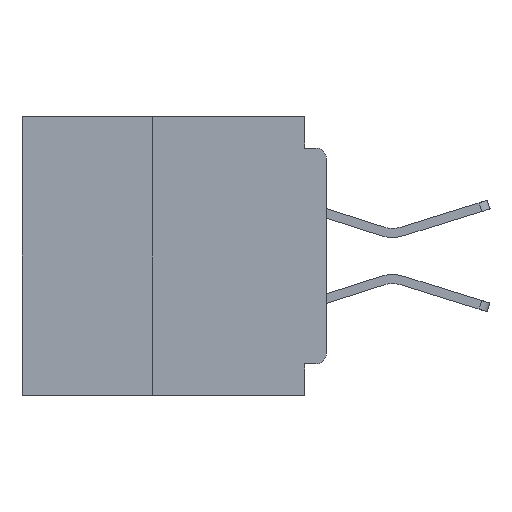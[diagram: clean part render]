
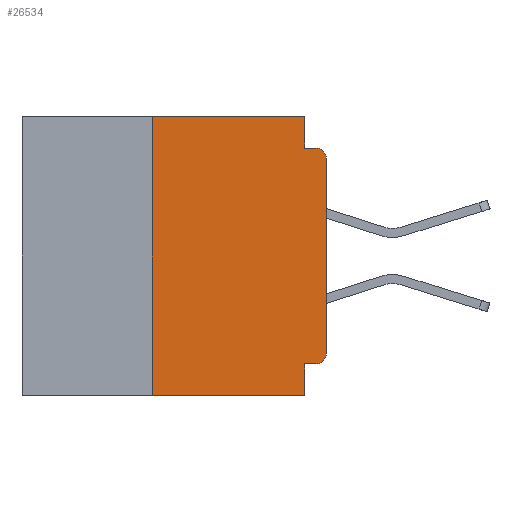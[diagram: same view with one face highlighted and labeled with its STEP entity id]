
A CAD part, left-side view. The second image highlights one B-rep face of the part: STEP entity #26534.
In plain terms, the highlighted planar face has unit normal (-1, 0, 0).
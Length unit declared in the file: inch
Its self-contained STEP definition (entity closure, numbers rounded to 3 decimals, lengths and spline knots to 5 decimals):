
#255 = CARTESIAN_POINT ( 'NONE',  ( 0., 0.437, -0.4 ) ) ;
#380 = AXIS2_PLACEMENT_3D ( 'NONE', #38324, #18297, #41635 ) ;
#1920 = ORIENTED_EDGE ( 'NONE', *, *, #42422, .T. ) ;
#1972 = VECTOR ( 'NONE', #17697, 39.37008 ) ;
#2018 = ORIENTED_EDGE ( 'NONE', *, *, #5475, .F. ) ;
#2225 = CIRCLE ( 'NONE', #36719, 0.015 ) ;
#2413 = EDGE_CURVE ( 'NONE', #28205, #35702, #32379, .T. ) ;
#3160 = CARTESIAN_POINT ( 'NONE',  ( 0., 0.015, -0.045 ) ) ;
#3316 = CARTESIAN_POINT ( 'NONE',  ( 0., 0.015, -0.34 ) ) ;
#3603 = CARTESIAN_POINT ( 'NONE',  ( 0., 0.031, -0.045 ) ) ;
#4029 = VECTOR ( 'NONE', #32181, 39.37008 ) ;
#4201 = VECTOR ( 'NONE', #35936, 39.37008 ) ;
#4441 = VECTOR ( 'NONE', #23019, 39.37008 ) ;
#4959 = CARTESIAN_POINT ( 'NONE',  ( 0., 0.25, -0.4 ) ) ;
#5108 = DIRECTION ( 'NONE',  ( 0., 0., 1. ) ) ;
#5475 = EDGE_CURVE ( 'NONE', #24682, #28205, #11640, .T. ) ;
#5590 = EDGE_CURVE ( 'NONE', #29763, #23510, #11081, .T. ) ;
#5641 = CARTESIAN_POINT ( 'NONE',  ( 0., 0., 0. ) ) ;
#6730 = DIRECTION ( 'NONE',  ( 0., 0., -1. ) ) ;
#7589 = EDGE_CURVE ( 'NONE', #35250, #29763, #30915, .T. ) ;
#7740 = LINE ( 'NONE', #255, #26707 ) ;
#8879 = CARTESIAN_POINT ( 'NONE',  ( 0., 0.437, 0. ) ) ;
#10181 = DIRECTION ( 'NONE',  ( 0., -1., 0. ) ) ;
#10432 = DIRECTION ( 'NONE',  ( 0., -1., 0. ) ) ;
#11081 = LINE ( 'NONE', #34374, #1972 ) ;
#11315 = AXIS2_PLACEMENT_3D ( 'NONE', #8879, #35766, #15731 ) ;
#11640 = LINE ( 'NONE', #20490, #16378 ) ;
#12328 = PLANE ( 'NONE',  #11315 ) ;
#12780 = CIRCLE ( 'NONE', #380, 0.015 ) ;
#13079 = EDGE_CURVE ( 'NONE', #35702, #27366, #16376, .T. ) ;
#13273 = LINE ( 'NONE', #5641, #4201 ) ;
#14278 = CARTESIAN_POINT ( 'NONE',  ( 0., 0.031, 0. ) ) ;
#14629 = ORIENTED_EDGE ( 'NONE', *, *, #16336, .T. ) ;
#15011 = VECTOR ( 'NONE', #5108, 39.37008 ) ;
#15263 = ORIENTED_EDGE ( 'NONE', *, *, #5590, .F. ) ;
#15731 = DIRECTION ( 'NONE',  ( 0., 0., -1. ) ) ;
#15941 = CARTESIAN_POINT ( 'NONE',  ( 0., 0.031, -0.4 ) ) ;
#16336 = EDGE_CURVE ( 'NONE', #43265, #23510, #7740, .T. ) ;
#16376 = LINE ( 'NONE', #27648, #42979 ) ;
#16378 = VECTOR ( 'NONE', #10181, 39.37008 ) ;
#16476 = EDGE_LOOP ( 'NONE', ( #32818, #27047, #25469, #39860, #2018, #36787, #14629, #15263, #42514, #1920 ) ) ;
#17697 = DIRECTION ( 'NONE',  ( 0., 0., -1. ) ) ;
#18297 = DIRECTION ( 'NONE',  ( -1., 0., 0. ) ) ;
#20490 = CARTESIAN_POINT ( 'NONE',  ( 0., 0.437, 0. ) ) ;
#21223 = CARTESIAN_POINT ( 'NONE',  ( 0., 0.25, 0. ) ) ;
#21516 = CARTESIAN_POINT ( 'NONE',  ( 0., 0.015, -0.355 ) ) ;
#23019 = DIRECTION ( 'NONE',  ( 0., 0., -1. ) ) ;
#23227 = CARTESIAN_POINT ( 'NONE',  ( 0., 0.031, 0. ) ) ;
#23510 = VERTEX_POINT ( 'NONE', #15941 ) ;
#24682 = VERTEX_POINT ( 'NONE', #21223 ) ;
#24717 = EDGE_CURVE ( 'NONE', #40321, #27366, #12780, .T. ) ;
#25469 = ORIENTED_EDGE ( 'NONE', *, *, #13079, .F. ) ;
#26047 = EDGE_CURVE ( 'NONE', #36116, #40321, #13273, .T. ) ;
#26534 = ADVANCED_FACE ( 'NONE', ( #36800 ), #12328, .F. ) ;
#26707 = VECTOR ( 'NONE', #10432, 39.37008 ) ;
#26911 = DIRECTION ( 'NONE',  ( -1., 0., 0. ) ) ;
#27047 = ORIENTED_EDGE ( 'NONE', *, *, #24717, .T. ) ;
#27366 = VERTEX_POINT ( 'NONE', #3160 ) ;
#27648 = CARTESIAN_POINT ( 'NONE',  ( 0., 0., -0.045 ) ) ;
#28205 = VERTEX_POINT ( 'NONE', #14278 ) ;
#28786 = CARTESIAN_POINT ( 'NONE',  ( 0., 0., -0.355 ) ) ;
#29481 = CARTESIAN_POINT ( 'NONE',  ( 0., 0., -0.34 ) ) ;
#29763 = VERTEX_POINT ( 'NONE', #31153 ) ;
#30915 = LINE ( 'NONE', #28786, #4029 ) ;
#31024 = DIRECTION ( 'NONE',  ( 0., -1., 0. ) ) ;
#31153 = CARTESIAN_POINT ( 'NONE',  ( 0., 0.031, -0.355 ) ) ;
#32181 = DIRECTION ( 'NONE',  ( 0., 1., 0. ) ) ;
#32369 = CARTESIAN_POINT ( 'NONE',  ( 0., 0., -0.06 ) ) ;
#32379 = LINE ( 'NONE', #23227, #4441 ) ;
#32818 = ORIENTED_EDGE ( 'NONE', *, *, #26047, .T. ) ;
#33659 = EDGE_CURVE ( 'NONE', #43265, #24682, #41628, .T. ) ;
#34374 = CARTESIAN_POINT ( 'NONE',  ( 0., 0.031, -0.4 ) ) ;
#35250 = VERTEX_POINT ( 'NONE', #21516 ) ;
#35702 = VERTEX_POINT ( 'NONE', #3603 ) ;
#35766 = DIRECTION ( 'NONE',  ( 1., 0., 0. ) ) ;
#35936 = DIRECTION ( 'NONE',  ( 0., 0., 1. ) ) ;
#36116 = VERTEX_POINT ( 'NONE', #29481 ) ;
#36719 = AXIS2_PLACEMENT_3D ( 'NONE', #3316, #26911, #6730 ) ;
#36787 = ORIENTED_EDGE ( 'NONE', *, *, #33659, .F. ) ;
#36800 = FACE_OUTER_BOUND ( 'NONE', #16476, .T. ) ;
#37627 = CARTESIAN_POINT ( 'NONE',  ( 0., 0.25, -0.4 ) ) ;
#38324 = CARTESIAN_POINT ( 'NONE',  ( 0., 0.015, -0.06 ) ) ;
#39860 = ORIENTED_EDGE ( 'NONE', *, *, #2413, .F. ) ;
#40321 = VERTEX_POINT ( 'NONE', #32369 ) ;
#41628 = LINE ( 'NONE', #4959, #15011 ) ;
#41635 = DIRECTION ( 'NONE',  ( 0., 0., -1. ) ) ;
#42422 = EDGE_CURVE ( 'NONE', #35250, #36116, #2225, .T. ) ;
#42514 = ORIENTED_EDGE ( 'NONE', *, *, #7589, .F. ) ;
#42979 = VECTOR ( 'NONE', #31024, 39.37008 ) ;
#43265 = VERTEX_POINT ( 'NONE', #37627 ) ;
